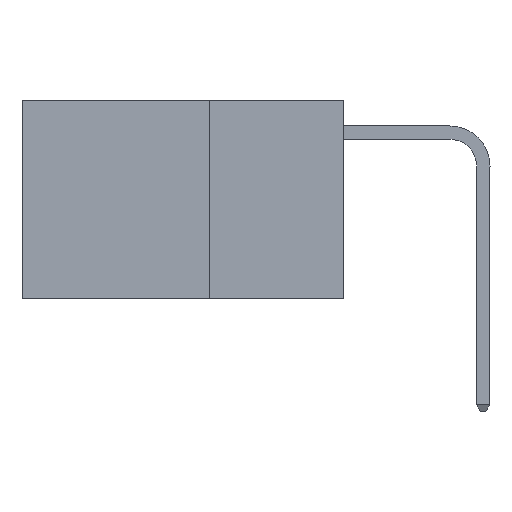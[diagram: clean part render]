
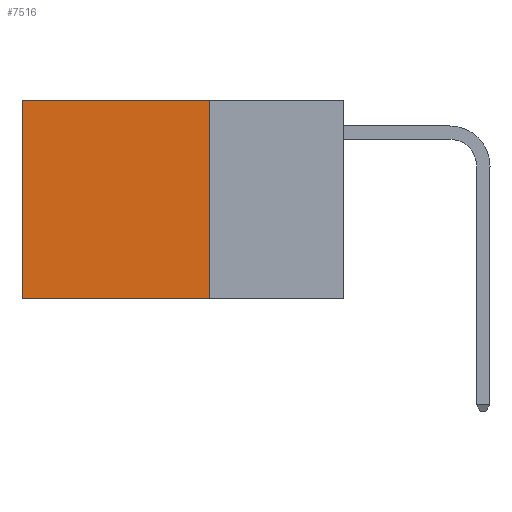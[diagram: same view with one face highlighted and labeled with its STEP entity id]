
A CAD part, left-side view. The second image highlights one B-rep face of the part: STEP entity #7516.
In plain terms, the highlighted planar face has unit normal (-1, 0, 0).
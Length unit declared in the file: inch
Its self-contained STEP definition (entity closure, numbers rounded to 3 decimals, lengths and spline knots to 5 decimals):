
#34 = DIRECTION ( 'NONE',  ( 0., 0., -1. ) ) ;
#566 = CARTESIAN_POINT ( 'NONE',  ( 0.2625, 0.6, -0.37 ) ) ;
#587 = LINE ( 'NONE', #1268, #904 ) ;
#904 = VECTOR ( 'NONE', #1328, 39.37008 ) ;
#1067 = DIRECTION ( 'NONE',  ( 0., 0., -1. ) ) ;
#1259 = PLANE ( 'NONE',  #8053 ) ;
#1268 = CARTESIAN_POINT ( 'NONE',  ( 0.2625, 0.6, 0. ) ) ;
#1317 = DIRECTION ( 'NONE',  ( 1., 0., 0. ) ) ;
#1328 = DIRECTION ( 'NONE',  ( 0., 0., -1. ) ) ;
#1446 = CARTESIAN_POINT ( 'NONE',  ( 0.2625, 0.25, 0. ) ) ;
#1531 = VERTEX_POINT ( 'NONE', #10853 ) ;
#2091 = ORIENTED_EDGE ( 'NONE', *, *, #5580, .F. ) ;
#2099 = DIRECTION ( 'NONE',  ( 0., 1., 0. ) ) ;
#2187 = VERTEX_POINT ( 'NONE', #3701 ) ;
#2489 = VERTEX_POINT ( 'NONE', #566 ) ;
#2984 = ORIENTED_EDGE ( 'NONE', *, *, #4982, .T. ) ;
#3701 = CARTESIAN_POINT ( 'NONE',  ( 0.2625, 0.6, 0. ) ) ;
#3833 = EDGE_LOOP ( 'NONE', ( #2984, #8934, #2091, #15049 ) ) ;
#4210 = FACE_OUTER_BOUND ( 'NONE', #3833, .T. ) ;
#4982 = EDGE_CURVE ( 'NONE', #2187, #2489, #587, .T. ) ;
#5580 = EDGE_CURVE ( 'NONE', #14375, #1531, #12623, .T. ) ;
#5611 = VECTOR ( 'NONE', #7205, 39.37008 ) ;
#5733 = LINE ( 'NONE', #6972, #5611 ) ;
#6972 = CARTESIAN_POINT ( 'NONE',  ( 0.2625, 0.25, -0.37 ) ) ;
#7184 = EDGE_CURVE ( 'NONE', #1531, #2489, #5733, .T. ) ;
#7205 = DIRECTION ( 'NONE',  ( 0., 1., 0. ) ) ;
#7516 = ADVANCED_FACE ( 'NONE', ( #4210 ), #1259, .F. ) ;
#7535 = CARTESIAN_POINT ( 'NONE',  ( 0.2625, 0.25, 0. ) ) ;
#7987 = CARTESIAN_POINT ( 'NONE',  ( 0.2625, 0.25, 0. ) ) ;
#8053 = AXIS2_PLACEMENT_3D ( 'NONE', #1446, #1317, #1067 ) ;
#8934 = ORIENTED_EDGE ( 'NONE', *, *, #7184, .F. ) ;
#9668 = VECTOR ( 'NONE', #2099, 39.37008 ) ;
#10137 = LINE ( 'NONE', #7987, #9668 ) ;
#10853 = CARTESIAN_POINT ( 'NONE',  ( 0.2625, 0.25, -0.37 ) ) ;
#12523 = VECTOR ( 'NONE', #34, 39.37008 ) ;
#12623 = LINE ( 'NONE', #14763, #12523 ) ;
#13526 = EDGE_CURVE ( 'NONE', #14375, #2187, #10137, .T. ) ;
#14375 = VERTEX_POINT ( 'NONE', #7535 ) ;
#14763 = CARTESIAN_POINT ( 'NONE',  ( 0.2625, 0.25, 0. ) ) ;
#15049 = ORIENTED_EDGE ( 'NONE', *, *, #13526, .T. ) ;
